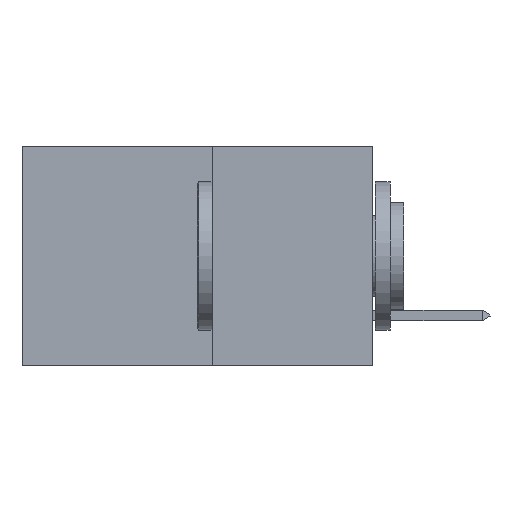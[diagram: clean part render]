
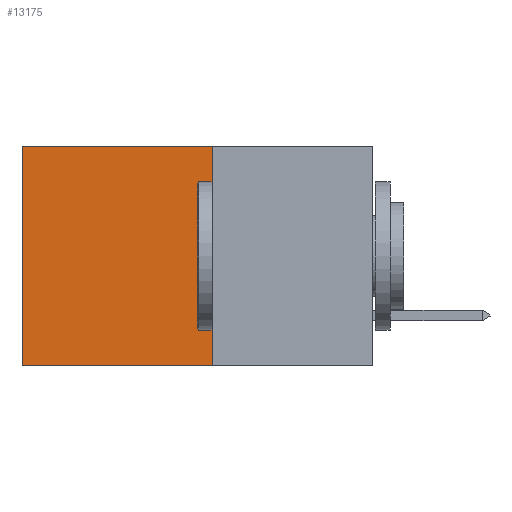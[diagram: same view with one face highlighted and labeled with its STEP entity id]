
A CAD part, left-side view. The second image highlights one B-rep face of the part: STEP entity #13175.
In plain terms, the highlighted planar face has unit normal (-1, 0, 0).
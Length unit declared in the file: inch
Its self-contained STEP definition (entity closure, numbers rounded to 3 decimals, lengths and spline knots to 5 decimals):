
#466 = DIRECTION ( 'NONE',  ( 0., 0., -1. ) ) ;
#527 = VERTEX_POINT ( 'NONE', #6510 ) ;
#2062 = EDGE_CURVE ( 'NONE', #7786, #3995, #5814, .T. ) ;
#2964 = CARTESIAN_POINT ( 'NONE',  ( 0.277, 0.27, -0.37 ) ) ;
#3950 = VECTOR ( 'NONE', #10054, 39.37008 ) ;
#3995 = VERTEX_POINT ( 'NONE', #14875 ) ;
#4413 = VECTOR ( 'NONE', #9947, 39.37008 ) ;
#4885 = CARTESIAN_POINT ( 'NONE',  ( 0.277, 0.27, 0. ) ) ;
#5729 = PLANE ( 'NONE',  #18115 ) ;
#5814 = LINE ( 'NONE', #13455, #10552 ) ;
#6510 = CARTESIAN_POINT ( 'NONE',  ( 0.277, 0.59, -0.37 ) ) ;
#7483 = VERTEX_POINT ( 'NONE', #14663 ) ;
#7530 = CARTESIAN_POINT ( 'NONE',  ( 0.277, 0.27, -0.37 ) ) ;
#7786 = VERTEX_POINT ( 'NONE', #4885 ) ;
#9313 = DIRECTION ( 'NONE',  ( 1., 0., 0. ) ) ;
#9947 = DIRECTION ( 'NONE',  ( 0., 1., 0. ) ) ;
#10054 = DIRECTION ( 'NONE',  ( 0., 1., 0. ) ) ;
#10091 = EDGE_CURVE ( 'NONE', #7786, #7483, #22755, .T. ) ;
#10552 = VECTOR ( 'NONE', #11041, 39.37008 ) ;
#11041 = DIRECTION ( 'NONE',  ( 0., 0., -1. ) ) ;
#13175 = ADVANCED_FACE ( 'NONE', ( #20404 ), #5729, .F. ) ;
#13251 = ORIENTED_EDGE ( 'NONE', *, *, #18266, .T. ) ;
#13455 = CARTESIAN_POINT ( 'NONE',  ( 0.277, 0.27, -0.37 ) ) ;
#14663 = CARTESIAN_POINT ( 'NONE',  ( 0.277, 0.59, 0. ) ) ;
#14875 = CARTESIAN_POINT ( 'NONE',  ( 0.277, 0.27, -0.37 ) ) ;
#15194 = ORIENTED_EDGE ( 'NONE', *, *, #2062, .F. ) ;
#16344 = EDGE_LOOP ( 'NONE', ( #13251, #21885, #15194, #22532 ) ) ;
#17301 = LINE ( 'NONE', #21702, #18414 ) ;
#18115 = AXIS2_PLACEMENT_3D ( 'NONE', #7530, #9313, #21701 ) ;
#18266 = EDGE_CURVE ( 'NONE', #7483, #527, #17301, .T. ) ;
#18414 = VECTOR ( 'NONE', #466, 39.37008 ) ;
#20361 = EDGE_CURVE ( 'NONE', #3995, #527, #22279, .T. ) ;
#20404 = FACE_OUTER_BOUND ( 'NONE', #16344, .T. ) ;
#20583 = CARTESIAN_POINT ( 'NONE',  ( 0.277, 0.27, 0. ) ) ;
#21701 = DIRECTION ( 'NONE',  ( 0., 0., -1. ) ) ;
#21702 = CARTESIAN_POINT ( 'NONE',  ( 0.277, 0.59, -0.37 ) ) ;
#21885 = ORIENTED_EDGE ( 'NONE', *, *, #20361, .F. ) ;
#22279 = LINE ( 'NONE', #2964, #3950 ) ;
#22532 = ORIENTED_EDGE ( 'NONE', *, *, #10091, .T. ) ;
#22755 = LINE ( 'NONE', #20583, #4413 ) ;
